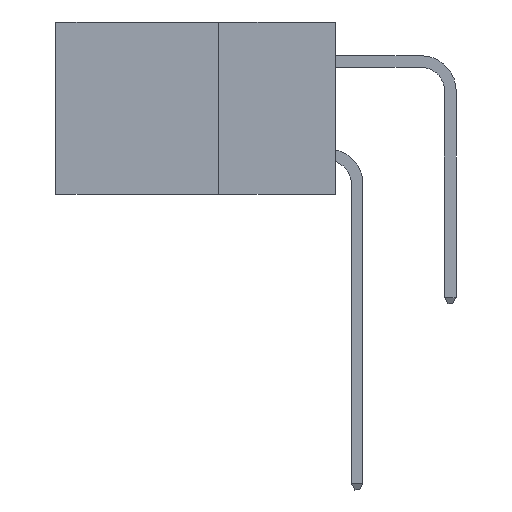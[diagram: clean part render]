
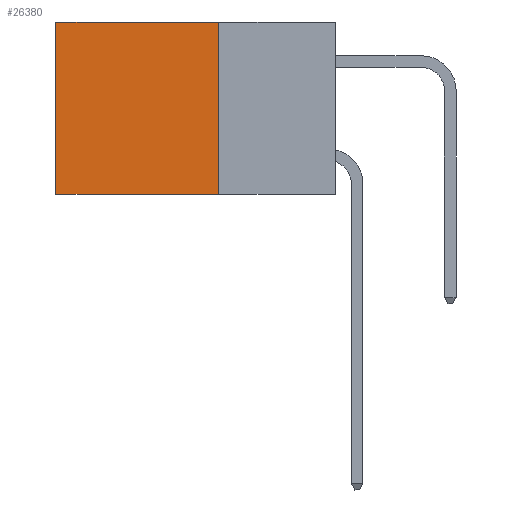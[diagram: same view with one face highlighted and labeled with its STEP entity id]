
A CAD part, left-side view. The second image highlights one B-rep face of the part: STEP entity #26380.
In plain terms, the highlighted planar face has unit normal (-1, 0, 0).
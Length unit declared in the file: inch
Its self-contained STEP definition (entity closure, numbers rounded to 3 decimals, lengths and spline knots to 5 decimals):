
#1717 = EDGE_CURVE ( 'NONE', #8877, #19017, #19158, .T. ) ;
#1770 = VECTOR ( 'NONE', #9727, 39.37008 ) ;
#4841 = DIRECTION ( 'NONE',  ( 0., 0., -1. ) ) ;
#6545 = VECTOR ( 'NONE', #26850, 39.37008 ) ;
#7299 = ORIENTED_EDGE ( 'NONE', *, *, #13630, .T. ) ;
#7522 = CARTESIAN_POINT ( 'NONE',  ( 0.2875, 0.25, 0. ) ) ;
#8634 = VERTEX_POINT ( 'NONE', #7522 ) ;
#8730 = LINE ( 'NONE', #19782, #15228 ) ;
#8830 = CARTESIAN_POINT ( 'NONE',  ( 0.2875, 0.6, 0. ) ) ;
#8877 = VERTEX_POINT ( 'NONE', #15110 ) ;
#9727 = DIRECTION ( 'NONE',  ( 0., 1., 0. ) ) ;
#9974 = ORIENTED_EDGE ( 'NONE', *, *, #25853, .F. ) ;
#10260 = FACE_OUTER_BOUND ( 'NONE', #21538, .T. ) ;
#10819 = DIRECTION ( 'NONE',  ( 0., 0., -1. ) ) ;
#12750 = LINE ( 'NONE', #29901, #6545 ) ;
#13630 = EDGE_CURVE ( 'NONE', #8634, #8877, #34857, .T. ) ;
#13689 = VERTEX_POINT ( 'NONE', #35201 ) ;
#15110 = CARTESIAN_POINT ( 'NONE',  ( 0.2875, 0.6, 0. ) ) ;
#15162 = ORIENTED_EDGE ( 'NONE', *, *, #16816, .F. ) ;
#15228 = VECTOR ( 'NONE', #22673, 39.37008 ) ;
#16816 = EDGE_CURVE ( 'NONE', #8634, #13689, #12750, .T. ) ;
#18289 = CARTESIAN_POINT ( 'NONE',  ( 0.2875, 0.6, -0.37 ) ) ;
#18592 = CARTESIAN_POINT ( 'NONE',  ( 0.2875, 0.25, 0. ) ) ;
#19017 = VERTEX_POINT ( 'NONE', #18289 ) ;
#19158 = LINE ( 'NONE', #8830, #26379 ) ;
#19782 = CARTESIAN_POINT ( 'NONE',  ( 0.2875, 0.25, -0.37 ) ) ;
#21538 = EDGE_LOOP ( 'NONE', ( #28379, #9974, #15162, #7299 ) ) ;
#22673 = DIRECTION ( 'NONE',  ( 0., 1., 0. ) ) ;
#24182 = CARTESIAN_POINT ( 'NONE',  ( 0.2875, 0.25, 0. ) ) ;
#25853 = EDGE_CURVE ( 'NONE', #13689, #19017, #8730, .T. ) ;
#26379 = VECTOR ( 'NONE', #10819, 39.37008 ) ;
#26380 = ADVANCED_FACE ( 'NONE', ( #10260 ), #26544, .F. ) ;
#26544 = PLANE ( 'NONE',  #30231 ) ;
#26850 = DIRECTION ( 'NONE',  ( 0., 0., -1. ) ) ;
#28379 = ORIENTED_EDGE ( 'NONE', *, *, #1717, .T. ) ;
#29095 = DIRECTION ( 'NONE',  ( 1., 0., 0. ) ) ;
#29901 = CARTESIAN_POINT ( 'NONE',  ( 0.2875, 0.25, 0. ) ) ;
#30231 = AXIS2_PLACEMENT_3D ( 'NONE', #24182, #29095, #4841 ) ;
#34857 = LINE ( 'NONE', #18592, #1770 ) ;
#35201 = CARTESIAN_POINT ( 'NONE',  ( 0.2875, 0.25, -0.37 ) ) ;
